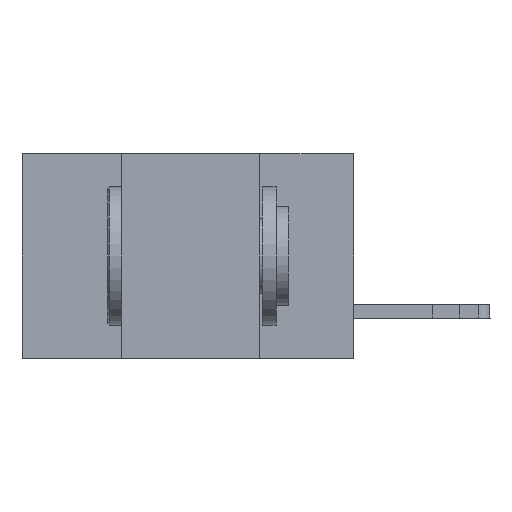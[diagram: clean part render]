
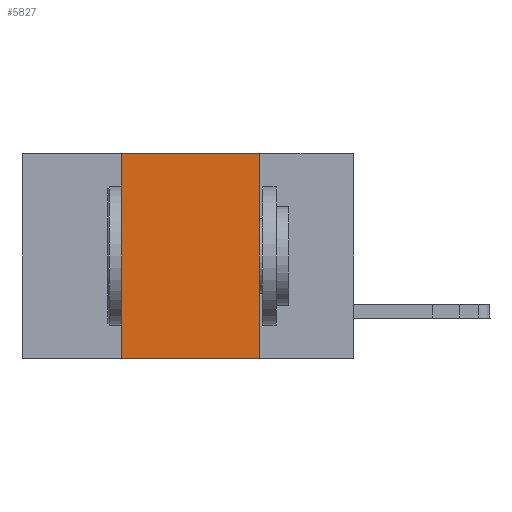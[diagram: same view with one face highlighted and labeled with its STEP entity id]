
A CAD part, left-side view. The second image highlights one B-rep face of the part: STEP entity #5827.
In plain terms, the highlighted planar face has unit normal (-1, 0, 0).
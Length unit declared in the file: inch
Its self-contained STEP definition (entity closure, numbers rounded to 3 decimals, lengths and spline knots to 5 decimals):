
#707 = DIRECTION ( 'NONE',  ( 0., 0., 1. ) ) ;
#1502 = EDGE_CURVE ( 'NONE', #20831, #21222, #8840, .T. ) ;
#1854 = DIRECTION ( 'NONE',  ( 0., 0., -1. ) ) ;
#1876 = EDGE_CURVE ( 'NONE', #20831, #13585, #15652, .T. ) ;
#2190 = VECTOR ( 'NONE', #7286, 39.37008 ) ;
#3920 = CARTESIAN_POINT ( 'NONE',  ( 0., 0.6, 0. ) ) ;
#4268 = ORIENTED_EDGE ( 'NONE', *, *, #21809, .F. ) ;
#5129 = LINE ( 'NONE', #7511, #13820 ) ;
#5475 = FACE_OUTER_BOUND ( 'NONE', #11188, .T. ) ;
#5827 = ADVANCED_FACE ( 'NONE', ( #5475 ), #26216, .F. ) ;
#6974 = VECTOR ( 'NONE', #14792, 39.37008 ) ;
#7286 = DIRECTION ( 'NONE',  ( 0., -1., 0. ) ) ;
#7511 = CARTESIAN_POINT ( 'NONE',  ( 0., 0.6, 0. ) ) ;
#8840 = LINE ( 'NONE', #21474, #11969 ) ;
#11188 = EDGE_LOOP ( 'NONE', ( #30014, #4268, #18744, #21303 ) ) ;
#11969 = VECTOR ( 'NONE', #707, 39.37008 ) ;
#13585 = VERTEX_POINT ( 'NONE', #26638 ) ;
#13820 = VECTOR ( 'NONE', #15532, 39.37008 ) ;
#14638 = LINE ( 'NONE', #19911, #6974 ) ;
#14792 = DIRECTION ( 'NONE',  ( 0., 0., -1. ) ) ;
#15532 = DIRECTION ( 'NONE',  ( 0., -1., 0. ) ) ;
#15652 = LINE ( 'NONE', #31261, #2190 ) ;
#17621 = EDGE_CURVE ( 'NONE', #25480, #13585, #14638, .T. ) ;
#18744 = ORIENTED_EDGE ( 'NONE', *, *, #1502, .F. ) ;
#19753 = DIRECTION ( 'NONE',  ( 1., 0., 0. ) ) ;
#19871 = CARTESIAN_POINT ( 'NONE',  ( 0., 0.42, -0.37 ) ) ;
#19911 = CARTESIAN_POINT ( 'NONE',  ( 0., 0.17, 0. ) ) ;
#20831 = VERTEX_POINT ( 'NONE', #19871 ) ;
#21222 = VERTEX_POINT ( 'NONE', #22202 ) ;
#21303 = ORIENTED_EDGE ( 'NONE', *, *, #1876, .T. ) ;
#21474 = CARTESIAN_POINT ( 'NONE',  ( 0., 0.42, 0. ) ) ;
#21809 = EDGE_CURVE ( 'NONE', #21222, #25480, #5129, .T. ) ;
#22202 = CARTESIAN_POINT ( 'NONE',  ( 0., 0.42, 0. ) ) ;
#25480 = VERTEX_POINT ( 'NONE', #28772 ) ;
#26216 = PLANE ( 'NONE',  #31687 ) ;
#26638 = CARTESIAN_POINT ( 'NONE',  ( 0., 0.17, -0.37 ) ) ;
#28772 = CARTESIAN_POINT ( 'NONE',  ( 0., 0.17, 0. ) ) ;
#30014 = ORIENTED_EDGE ( 'NONE', *, *, #17621, .F. ) ;
#31261 = CARTESIAN_POINT ( 'NONE',  ( 0., 0.6, -0.37 ) ) ;
#31687 = AXIS2_PLACEMENT_3D ( 'NONE', #3920, #19753, #1854 ) ;
